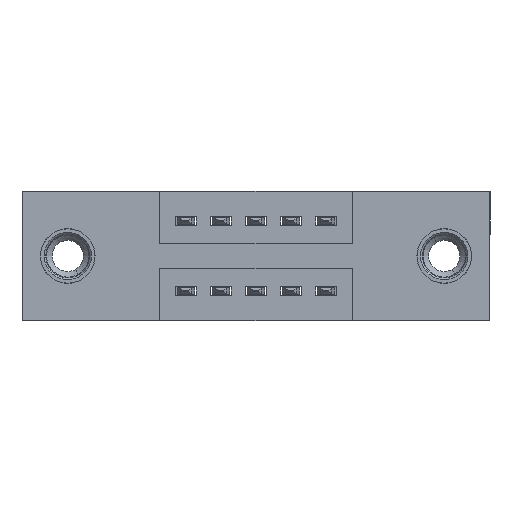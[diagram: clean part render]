
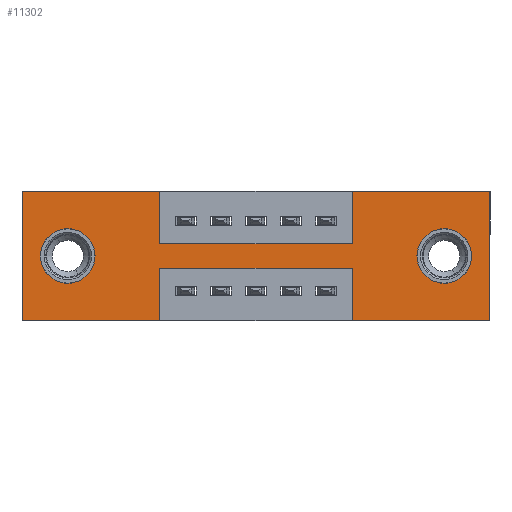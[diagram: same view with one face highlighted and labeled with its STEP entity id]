
A CAD part, front view. The second image highlights one B-rep face of the part: STEP entity #11302.
In plain terms, the highlighted planar face has unit normal (0, -1, 0).
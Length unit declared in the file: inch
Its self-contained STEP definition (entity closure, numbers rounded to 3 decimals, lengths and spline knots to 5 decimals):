
#111 = VERTEX_POINT ( 'NONE', #5772 ) ;
#150 = DIRECTION ( 'NONE',  ( 0., 0., -1. ) ) ;
#187 = CARTESIAN_POINT ( 'NONE',  ( 1.205, 0., -0.185 ) ) ;
#212 = VERTEX_POINT ( 'NONE', #5248 ) ;
#292 = CARTESIAN_POINT ( 'NONE',  ( 0., 0., -0.37 ) ) ;
#336 = VERTEX_POINT ( 'NONE', #5812 ) ;
#571 = VECTOR ( 'NONE', #150, 39.37008 ) ;
#589 = CARTESIAN_POINT ( 'NONE',  ( 1.205, 0., -0.107 ) ) ;
#736 = VECTOR ( 'NONE', #8555, 39.37008 ) ;
#784 = EDGE_CURVE ( 'NONE', #8121, #5027, #3291, .T. ) ;
#897 = ORIENTED_EDGE ( 'NONE', *, *, #8018, .T. ) ;
#1244 = DIRECTION ( 'NONE',  ( 0., 0., -1. ) ) ;
#1274 = EDGE_CURVE ( 'NONE', #12472, #2052, #8090, .T. ) ;
#1362 = CARTESIAN_POINT ( 'NONE',  ( 0., 0., 0. ) ) ;
#1712 = CARTESIAN_POINT ( 'NONE',  ( 0., 0., 0. ) ) ;
#1722 = EDGE_CURVE ( 'NONE', #111, #12881, #5074, .T. ) ;
#2052 = VERTEX_POINT ( 'NONE', #2245 ) ;
#2056 = CARTESIAN_POINT ( 'NONE',  ( 0.9425, 0., 0. ) ) ;
#2245 = CARTESIAN_POINT ( 'NONE',  ( 0.3925, 0., -0.15 ) ) ;
#2348 = FACE_OUTER_BOUND ( 'NONE', #6341, .T. ) ;
#2468 = DIRECTION ( 'NONE',  ( 0., 0., 1. ) ) ;
#2665 = EDGE_CURVE ( 'NONE', #5754, #13783, #12720, .T. ) ;
#2751 = DIRECTION ( 'NONE',  ( 0., 0., -1. ) ) ;
#2866 = ORIENTED_EDGE ( 'NONE', *, *, #13801, .F. ) ;
#3009 = CARTESIAN_POINT ( 'NONE',  ( 0.13, 0., -0.263 ) ) ;
#3037 = AXIS2_PLACEMENT_3D ( 'NONE', #3134, #12661, #6279 ) ;
#3109 = LINE ( 'NONE', #4822, #9106 ) ;
#3134 = CARTESIAN_POINT ( 'NONE',  ( 0.13, 0., -0.185 ) ) ;
#3145 = ORIENTED_EDGE ( 'NONE', *, *, #10544, .F. ) ;
#3214 = LINE ( 'NONE', #4366, #571 ) ;
#3291 = LINE ( 'NONE', #7708, #6454 ) ;
#3488 = VERTEX_POINT ( 'NONE', #4642 ) ;
#3497 = FACE_BOUND ( 'NONE', #11532, .T. ) ;
#3500 = EDGE_CURVE ( 'NONE', #13319, #12472, #9849, .T. ) ;
#3703 = EDGE_CURVE ( 'NONE', #5027, #8528, #8150, .T. ) ;
#4015 = EDGE_CURVE ( 'NONE', #6238, #8121, #9499, .T. ) ;
#4100 = CARTESIAN_POINT ( 'NONE',  ( 0.3925, 0., -0.22 ) ) ;
#4219 = CARTESIAN_POINT ( 'NONE',  ( 0., 0., -0.37 ) ) ;
#4332 = ORIENTED_EDGE ( 'NONE', *, *, #4015, .F. ) ;
#4366 = CARTESIAN_POINT ( 'NONE',  ( 1.335, 0., 0. ) ) ;
#4554 = DIRECTION ( 'NONE',  ( 0., 1., 0. ) ) ;
#4592 = CARTESIAN_POINT ( 'NONE',  ( 0.3925, 0., -0.15 ) ) ;
#4642 = CARTESIAN_POINT ( 'NONE',  ( 0.9425, 0., -0.15 ) ) ;
#4681 = DIRECTION ( 'NONE',  ( 1., 0., 0. ) ) ;
#4781 = CARTESIAN_POINT ( 'NONE',  ( 1.205, 0., -0.263 ) ) ;
#4822 = CARTESIAN_POINT ( 'NONE',  ( 0.3925, 0., -0.37 ) ) ;
#4911 = DIRECTION ( 'NONE',  ( 0., 0., -1. ) ) ;
#5027 = VERTEX_POINT ( 'NONE', #8925 ) ;
#5074 = CIRCLE ( 'NONE', #3037, 0.078 ) ;
#5248 = CARTESIAN_POINT ( 'NONE',  ( 0., 0., -0.37 ) ) ;
#5281 = VECTOR ( 'NONE', #13015, 39.37008 ) ;
#5295 = DIRECTION ( 'NONE',  ( 0., 1., 0. ) ) ;
#5444 = DIRECTION ( 'NONE',  ( 0., 1., 0. ) ) ;
#5539 = CIRCLE ( 'NONE', #7893, 0.078 ) ;
#5559 = DIRECTION ( 'NONE',  ( 0., 0., 1. ) ) ;
#5674 = ORIENTED_EDGE ( 'NONE', *, *, #3703, .F. ) ;
#5695 = LINE ( 'NONE', #10815, #736 ) ;
#5754 = VERTEX_POINT ( 'NONE', #4781 ) ;
#5772 = CARTESIAN_POINT ( 'NONE',  ( 0.13, 0., -0.107 ) ) ;
#5812 = CARTESIAN_POINT ( 'NONE',  ( 1.335, 0., 0. ) ) ;
#6238 = VERTEX_POINT ( 'NONE', #9076 ) ;
#6279 = DIRECTION ( 'NONE',  ( 0., 0., 1. ) ) ;
#6337 = CARTESIAN_POINT ( 'NONE',  ( 0., 0., 0. ) ) ;
#6341 = EDGE_LOOP ( 'NONE', ( #2866, #5674, #11259, #4332, #12583, #11639, #10285, #12779, #11919, #10922, #3145, #11216 ) ) ;
#6373 = DIRECTION ( 'NONE',  ( 0., 0., -1. ) ) ;
#6454 = VECTOR ( 'NONE', #5559, 39.37008 ) ;
#6466 = PLANE ( 'NONE',  #7831 ) ;
#6502 = DIRECTION ( 'NONE',  ( -1., 0., 0. ) ) ;
#6520 = CARTESIAN_POINT ( 'NONE',  ( 0.9425, 0., -0.37 ) ) ;
#6593 = VERTEX_POINT ( 'NONE', #8875 ) ;
#7013 = VECTOR ( 'NONE', #10929, 39.37008 ) ;
#7147 = ORIENTED_EDGE ( 'NONE', *, *, #2665, .T. ) ;
#7415 = EDGE_LOOP ( 'NONE', ( #10325, #13618 ) ) ;
#7528 = CARTESIAN_POINT ( 'NONE',  ( 0., 0., -0.37 ) ) ;
#7530 = CARTESIAN_POINT ( 'NONE',  ( 1.205, 0., -0.185 ) ) ;
#7708 = CARTESIAN_POINT ( 'NONE',  ( 0.9425, 0., -0.37 ) ) ;
#7822 = VECTOR ( 'NONE', #11248, 39.37008 ) ;
#7831 = AXIS2_PLACEMENT_3D ( 'NONE', #7528, #12886, #10744 ) ;
#7893 = AXIS2_PLACEMENT_3D ( 'NONE', #7530, #5295, #6373 ) ;
#7931 = AXIS2_PLACEMENT_3D ( 'NONE', #187, #5444, #1244 ) ;
#8018 = EDGE_CURVE ( 'NONE', #13783, #5754, #5539, .T. ) ;
#8090 = LINE ( 'NONE', #10144, #10917 ) ;
#8107 = DIRECTION ( 'NONE',  ( 0., 0., 1. ) ) ;
#8121 = VERTEX_POINT ( 'NONE', #6520 ) ;
#8150 = LINE ( 'NONE', #11203, #7822 ) ;
#8303 = LINE ( 'NONE', #8837, #5281 ) ;
#8528 = VERTEX_POINT ( 'NONE', #4100 ) ;
#8555 = DIRECTION ( 'NONE',  ( 1., 0., 0. ) ) ;
#8561 = EDGE_CURVE ( 'NONE', #336, #6238, #3214, .T. ) ;
#8597 = EDGE_CURVE ( 'NONE', #11911, #336, #5695, .T. ) ;
#8837 = CARTESIAN_POINT ( 'NONE',  ( 0.9425, 0., 0. ) ) ;
#8875 = CARTESIAN_POINT ( 'NONE',  ( 0.3925, 0., -0.37 ) ) ;
#8883 = CARTESIAN_POINT ( 'NONE',  ( 0.3925, 0., 0. ) ) ;
#8898 = CARTESIAN_POINT ( 'NONE',  ( 0.13, 0., -0.185 ) ) ;
#8925 = CARTESIAN_POINT ( 'NONE',  ( 0.9425, 0., -0.22 ) ) ;
#9076 = CARTESIAN_POINT ( 'NONE',  ( 1.335, 0., -0.37 ) ) ;
#9106 = VECTOR ( 'NONE', #4911, 39.37008 ) ;
#9277 = EDGE_CURVE ( 'NONE', #12881, #111, #12173, .T. ) ;
#9499 = LINE ( 'NONE', #292, #13333 ) ;
#9507 = FACE_BOUND ( 'NONE', #7415, .T. ) ;
#9849 = LINE ( 'NONE', #1362, #7013 ) ;
#10144 = CARTESIAN_POINT ( 'NONE',  ( 0.3925, 0., 0. ) ) ;
#10285 = ORIENTED_EDGE ( 'NONE', *, *, #12395, .F. ) ;
#10325 = ORIENTED_EDGE ( 'NONE', *, *, #1722, .T. ) ;
#10544 = EDGE_CURVE ( 'NONE', #212, #13319, #11676, .T. ) ;
#10582 = DIRECTION ( 'NONE',  ( -1., 0., 0. ) ) ;
#10744 = DIRECTION ( 'NONE',  ( 0., 0., -1. ) ) ;
#10815 = CARTESIAN_POINT ( 'NONE',  ( 0., 0., 0. ) ) ;
#10917 = VECTOR ( 'NONE', #2751, 39.37008 ) ;
#10922 = ORIENTED_EDGE ( 'NONE', *, *, #3500, .F. ) ;
#10929 = DIRECTION ( 'NONE',  ( 1., 0., 0. ) ) ;
#11203 = CARTESIAN_POINT ( 'NONE',  ( 0.3925, 0., -0.22 ) ) ;
#11216 = ORIENTED_EDGE ( 'NONE', *, *, #12764, .F. ) ;
#11248 = DIRECTION ( 'NONE',  ( -1., 0., 0. ) ) ;
#11259 = ORIENTED_EDGE ( 'NONE', *, *, #784, .F. ) ;
#11302 = ADVANCED_FACE ( 'NONE', ( #3497, #9507, #2348 ), #6466, .T. ) ;
#11441 = EDGE_CURVE ( 'NONE', #2052, #3488, #12825, .T. ) ;
#11450 = VECTOR ( 'NONE', #10582, 39.37008 ) ;
#11532 = EDGE_LOOP ( 'NONE', ( #897, #7147 ) ) ;
#11639 = ORIENTED_EDGE ( 'NONE', *, *, #8597, .F. ) ;
#11676 = LINE ( 'NONE', #1712, #13528 ) ;
#11911 = VERTEX_POINT ( 'NONE', #2056 ) ;
#11919 = ORIENTED_EDGE ( 'NONE', *, *, #1274, .F. ) ;
#11972 = VECTOR ( 'NONE', #4681, 39.37008 ) ;
#12173 = CIRCLE ( 'NONE', #12275, 0.078 ) ;
#12275 = AXIS2_PLACEMENT_3D ( 'NONE', #8898, #4554, #2468 ) ;
#12276 = LINE ( 'NONE', #4219, #11450 ) ;
#12395 = EDGE_CURVE ( 'NONE', #3488, #11911, #8303, .T. ) ;
#12472 = VERTEX_POINT ( 'NONE', #8883 ) ;
#12583 = ORIENTED_EDGE ( 'NONE', *, *, #8561, .F. ) ;
#12661 = DIRECTION ( 'NONE',  ( 0., 1., 0. ) ) ;
#12720 = CIRCLE ( 'NONE', #7931, 0.078 ) ;
#12764 = EDGE_CURVE ( 'NONE', #6593, #212, #12276, .T. ) ;
#12779 = ORIENTED_EDGE ( 'NONE', *, *, #11441, .F. ) ;
#12825 = LINE ( 'NONE', #4592, #11972 ) ;
#12881 = VERTEX_POINT ( 'NONE', #3009 ) ;
#12886 = DIRECTION ( 'NONE',  ( 0., -1., 0. ) ) ;
#13015 = DIRECTION ( 'NONE',  ( 0., 0., 1. ) ) ;
#13319 = VERTEX_POINT ( 'NONE', #6337 ) ;
#13333 = VECTOR ( 'NONE', #6502, 39.37008 ) ;
#13528 = VECTOR ( 'NONE', #8107, 39.37008 ) ;
#13618 = ORIENTED_EDGE ( 'NONE', *, *, #9277, .T. ) ;
#13783 = VERTEX_POINT ( 'NONE', #589 ) ;
#13801 = EDGE_CURVE ( 'NONE', #8528, #6593, #3109, .T. ) ;
